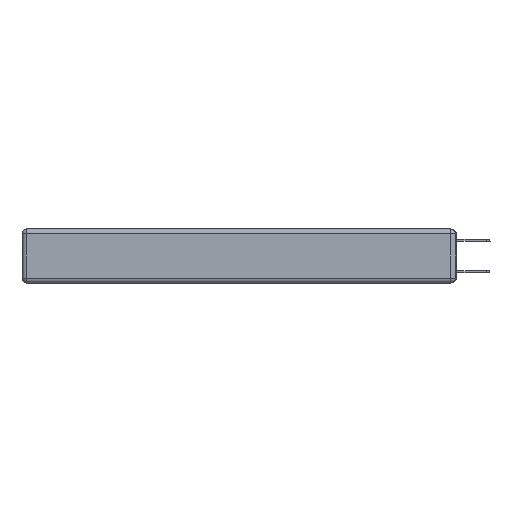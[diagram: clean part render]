
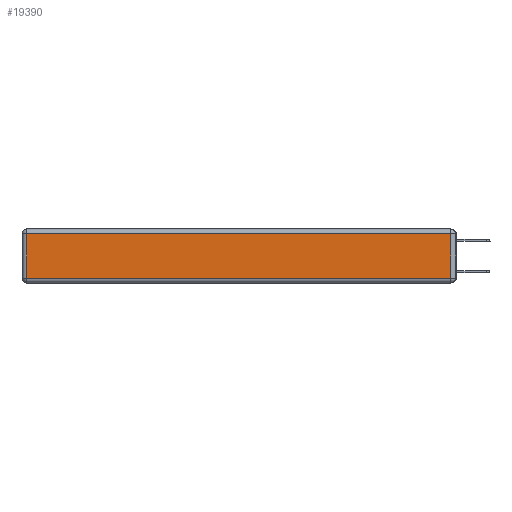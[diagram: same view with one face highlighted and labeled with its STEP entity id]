
A CAD part, left-side view. The second image highlights one B-rep face of the part: STEP entity #19390.
In plain terms, the highlighted planar face has unit normal (-1, 0, 0).
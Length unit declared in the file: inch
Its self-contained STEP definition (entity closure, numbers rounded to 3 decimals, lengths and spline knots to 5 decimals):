
#238 = ORIENTED_EDGE ( 'NONE', *, *, #20845, .T. ) ;
#259 = CARTESIAN_POINT ( 'NONE',  ( 0., 2.72, -0.03 ) ) ;
#528 = CARTESIAN_POINT ( 'NONE',  ( 0., 0., -0.313 ) ) ;
#1330 = DIRECTION ( 'NONE',  ( 0., 1., 0. ) ) ;
#2050 = CARTESIAN_POINT ( 'NONE',  ( 0., 0.03, -0.343 ) ) ;
#5058 = DIRECTION ( 'NONE',  ( 0., 0., 1. ) ) ;
#5386 = CARTESIAN_POINT ( 'NONE',  ( 0., 0.03, -0.313 ) ) ;
#6216 = LINE ( 'NONE', #528, #14618 ) ;
#6513 = VERTEX_POINT ( 'NONE', #23583 ) ;
#6787 = CARTESIAN_POINT ( 'NONE',  ( 0., 2.72, -0.343 ) ) ;
#7855 = CARTESIAN_POINT ( 'NONE',  ( 0., 2.75, -0.03 ) ) ;
#8452 = DIRECTION ( 'NONE',  ( 0., 0., 1. ) ) ;
#8496 = ORIENTED_EDGE ( 'NONE', *, *, #21828, .T. ) ;
#10421 = LINE ( 'NONE', #2050, #24849 ) ;
#11532 = FACE_OUTER_BOUND ( 'NONE', #16294, .T. ) ;
#11632 = PLANE ( 'NONE',  #18792 ) ;
#11763 = VERTEX_POINT ( 'NONE', #5386 ) ;
#13209 = EDGE_CURVE ( 'NONE', #14859, #25115, #22500, .T. ) ;
#13500 = DIRECTION ( 'NONE',  ( 0., -1., 0. ) ) ;
#14618 = VECTOR ( 'NONE', #13500, 39.37008 ) ;
#14859 = VERTEX_POINT ( 'NONE', #22127 ) ;
#16294 = EDGE_LOOP ( 'NONE', ( #22643, #238, #22777, #8496 ) ) ;
#17597 = DIRECTION ( 'NONE',  ( 0., 0., -1. ) ) ;
#17914 = DIRECTION ( 'NONE',  ( -1., 0., 0. ) ) ;
#18792 = AXIS2_PLACEMENT_3D ( 'NONE', #26458, #17914, #5058 ) ;
#19390 = ADVANCED_FACE ( 'NONE', ( #11532 ), #11632, .T. ) ;
#19765 = LINE ( 'NONE', #6787, #25793 ) ;
#19801 = VECTOR ( 'NONE', #1330, 39.37008 ) ;
#20845 = EDGE_CURVE ( 'NONE', #11763, #14859, #10421, .T. ) ;
#21828 = EDGE_CURVE ( 'NONE', #25115, #6513, #19765, .T. ) ;
#22127 = CARTESIAN_POINT ( 'NONE',  ( 0., 0.03, -0.03 ) ) ;
#22500 = LINE ( 'NONE', #7855, #19801 ) ;
#22643 = ORIENTED_EDGE ( 'NONE', *, *, #24518, .T. ) ;
#22777 = ORIENTED_EDGE ( 'NONE', *, *, #13209, .T. ) ;
#23583 = CARTESIAN_POINT ( 'NONE',  ( 0., 2.72, -0.313 ) ) ;
#24518 = EDGE_CURVE ( 'NONE', #6513, #11763, #6216, .T. ) ;
#24849 = VECTOR ( 'NONE', #8452, 39.37008 ) ;
#25115 = VERTEX_POINT ( 'NONE', #259 ) ;
#25793 = VECTOR ( 'NONE', #17597, 39.37008 ) ;
#26458 = CARTESIAN_POINT ( 'NONE',  ( 0., 0., -0.343 ) ) ;
